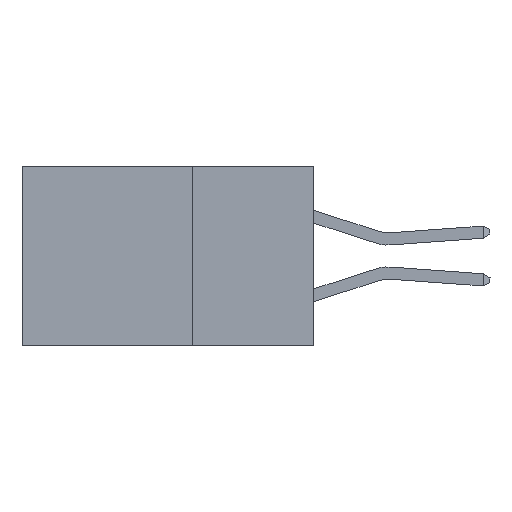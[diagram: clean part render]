
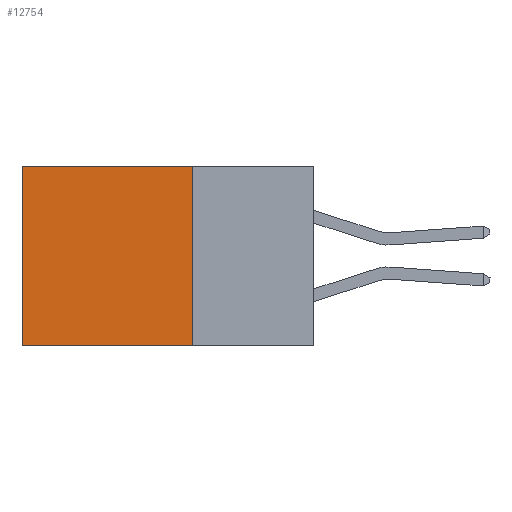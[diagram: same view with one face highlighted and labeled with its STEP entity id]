
A CAD part, left-side view. The second image highlights one B-rep face of the part: STEP entity #12754.
In plain terms, the highlighted planar face has unit normal (-1, 0, 0).
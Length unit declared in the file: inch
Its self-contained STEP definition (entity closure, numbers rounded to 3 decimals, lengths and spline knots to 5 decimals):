
#66 = CARTESIAN_POINT ( 'NONE',  ( 0.2875, 0.25, -0.37 ) ) ;
#274 = DIRECTION ( 'NONE',  ( 0., 1., 0. ) ) ;
#603 = ORIENTED_EDGE ( 'NONE', *, *, #10419, .T. ) ;
#882 = DIRECTION ( 'NONE',  ( 0., 0., -1. ) ) ;
#1457 = CARTESIAN_POINT ( 'NONE',  ( 0.2875, 0.25, 0. ) ) ;
#1948 = EDGE_CURVE ( 'NONE', #14604, #8118, #12800, .T. ) ;
#2494 = DIRECTION ( 'NONE',  ( 0., 0., -1. ) ) ;
#2589 = VERTEX_POINT ( 'NONE', #1457 ) ;
#2884 = EDGE_CURVE ( 'NONE', #2589, #10701, #13162, .T. ) ;
#2937 = DIRECTION ( 'NONE',  ( 0., 0., -1. ) ) ;
#3621 = LINE ( 'NONE', #6932, #10101 ) ;
#4639 = CARTESIAN_POINT ( 'NONE',  ( 0.2875, 0.25, -0.37 ) ) ;
#4956 = PLANE ( 'NONE',  #6834 ) ;
#6011 = ORIENTED_EDGE ( 'NONE', *, *, #2884, .T. ) ;
#6022 = ORIENTED_EDGE ( 'NONE', *, *, #1948, .F. ) ;
#6216 = CARTESIAN_POINT ( 'NONE',  ( 0.2875, 0.25, 0. ) ) ;
#6454 = VECTOR ( 'NONE', #274, 39.37008 ) ;
#6834 = AXIS2_PLACEMENT_3D ( 'NONE', #6216, #8858, #882 ) ;
#6932 = CARTESIAN_POINT ( 'NONE',  ( 0.2875, 0.6, 0. ) ) ;
#7049 = VECTOR ( 'NONE', #2494, 39.37008 ) ;
#7134 = CARTESIAN_POINT ( 'NONE',  ( 0.2875, 0.6, 0. ) ) ;
#8118 = VERTEX_POINT ( 'NONE', #12209 ) ;
#8858 = DIRECTION ( 'NONE',  ( 1., 0., 0. ) ) ;
#10044 = LINE ( 'NONE', #10307, #7049 ) ;
#10101 = VECTOR ( 'NONE', #2937, 39.37008 ) ;
#10307 = CARTESIAN_POINT ( 'NONE',  ( 0.2875, 0.25, 0. ) ) ;
#10419 = EDGE_CURVE ( 'NONE', #10701, #8118, #3621, .T. ) ;
#10701 = VERTEX_POINT ( 'NONE', #7134 ) ;
#11065 = EDGE_LOOP ( 'NONE', ( #603, #6022, #16664, #6011 ) ) ;
#12177 = EDGE_CURVE ( 'NONE', #2589, #14604, #10044, .T. ) ;
#12209 = CARTESIAN_POINT ( 'NONE',  ( 0.2875, 0.6, -0.37 ) ) ;
#12464 = DIRECTION ( 'NONE',  ( 0., 1., 0. ) ) ;
#12620 = CARTESIAN_POINT ( 'NONE',  ( 0.2875, 0.25, 0. ) ) ;
#12754 = ADVANCED_FACE ( 'NONE', ( #15541 ), #4956, .F. ) ;
#12766 = VECTOR ( 'NONE', #12464, 39.37008 ) ;
#12800 = LINE ( 'NONE', #66, #6454 ) ;
#13162 = LINE ( 'NONE', #12620, #12766 ) ;
#14604 = VERTEX_POINT ( 'NONE', #4639 ) ;
#15541 = FACE_OUTER_BOUND ( 'NONE', #11065, .T. ) ;
#16664 = ORIENTED_EDGE ( 'NONE', *, *, #12177, .F. ) ;
